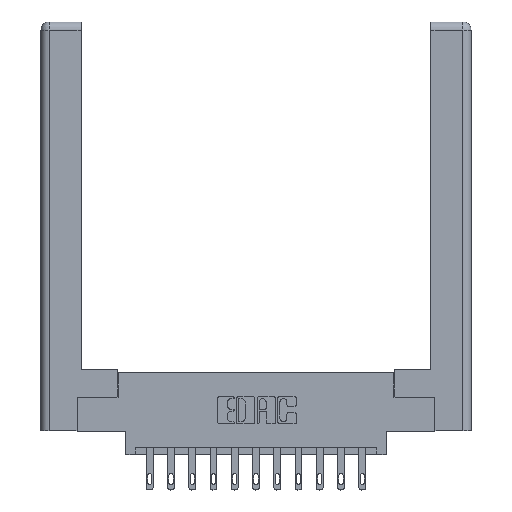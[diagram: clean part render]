
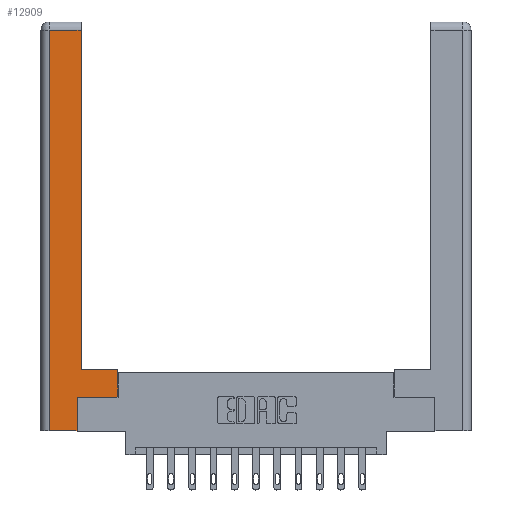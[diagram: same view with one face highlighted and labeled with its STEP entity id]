
A CAD part, top view. The second image highlights one B-rep face of the part: STEP entity #12909.
In plain terms, the highlighted planar face has unit normal (0, 0, 1).
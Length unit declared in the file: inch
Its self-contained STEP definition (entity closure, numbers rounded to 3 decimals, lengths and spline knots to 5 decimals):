
#191 = EDGE_CURVE ( 'NONE', #5089, #2664, #8265, .T. ) ;
#409 = CARTESIAN_POINT ( 'NONE',  ( 0.265, 0.245, 0. ) ) ;
#524 = CARTESIAN_POINT ( 'NONE',  ( 0.295, 2.94, 0. ) ) ;
#637 = DIRECTION ( 'NONE',  ( -1., 0., 0. ) ) ;
#660 = VECTOR ( 'NONE', #7658, 39.37008 ) ;
#1193 = VERTEX_POINT ( 'NONE', #10717 ) ;
#2319 = CARTESIAN_POINT ( 'NONE',  ( 0.565, 0.245, 0. ) ) ;
#2436 = VERTEX_POINT ( 'NONE', #524 ) ;
#2641 = DIRECTION ( 'NONE',  ( -1., 0., 0. ) ) ;
#2664 = VERTEX_POINT ( 'NONE', #14087 ) ;
#2863 = VECTOR ( 'NONE', #14801, 39.37008 ) ;
#3457 = EDGE_CURVE ( 'NONE', #7770, #2436, #3869, .T. ) ;
#3740 = CARTESIAN_POINT ( 'NONE',  ( 0.265, 0., 0. ) ) ;
#3869 = LINE ( 'NONE', #9389, #5882 ) ;
#4105 = EDGE_LOOP ( 'NONE', ( #7045, #4222, #13725, #10684, #13144, #4409, #6408, #6317 ) ) ;
#4153 = LINE ( 'NONE', #11201, #2863 ) ;
#4222 = ORIENTED_EDGE ( 'NONE', *, *, #10051, .T. ) ;
#4333 = EDGE_CURVE ( 'NONE', #14912, #11302, #10878, .T. ) ;
#4409 = ORIENTED_EDGE ( 'NONE', *, *, #7809, .T. ) ;
#4442 = DIRECTION ( 'NONE',  ( 0., 1., 0. ) ) ;
#4651 = VECTOR ( 'NONE', #6125, 39.37008 ) ;
#4731 = AXIS2_PLACEMENT_3D ( 'NONE', #11183, #9996, #637 ) ;
#4962 = CARTESIAN_POINT ( 'NONE',  ( 0.0615, 0., 0. ) ) ;
#4997 = CARTESIAN_POINT ( 'NONE',  ( 0.0615, 2.94, 0. ) ) ;
#5089 = VERTEX_POINT ( 'NONE', #9473 ) ;
#5126 = VECTOR ( 'NONE', #11988, 39.37008 ) ;
#5882 = VECTOR ( 'NONE', #10430, 39.37008 ) ;
#6070 = CARTESIAN_POINT ( 'NONE',  ( 0.295, 0.45, 0. ) ) ;
#6125 = DIRECTION ( 'NONE',  ( -1., 0., 0. ) ) ;
#6143 = LINE ( 'NONE', #2319, #7055 ) ;
#6317 = ORIENTED_EDGE ( 'NONE', *, *, #7481, .T. ) ;
#6408 = ORIENTED_EDGE ( 'NONE', *, *, #8894, .T. ) ;
#6705 = CARTESIAN_POINT ( 'NONE',  ( 0.265, 0.245, 0. ) ) ;
#6817 = VECTOR ( 'NONE', #4442, 39.37008 ) ;
#6964 = EDGE_CURVE ( 'NONE', #2664, #14912, #4153, .T. ) ;
#7045 = ORIENTED_EDGE ( 'NONE', *, *, #3457, .T. ) ;
#7055 = VECTOR ( 'NONE', #11638, 39.37008 ) ;
#7118 = VERTEX_POINT ( 'NONE', #11609 ) ;
#7481 = EDGE_CURVE ( 'NONE', #1193, #7770, #10954, .T. ) ;
#7658 = DIRECTION ( 'NONE',  ( 0., 1., 0. ) ) ;
#7667 = PLANE ( 'NONE',  #4731 ) ;
#7770 = VERTEX_POINT ( 'NONE', #13946 ) ;
#7809 = EDGE_CURVE ( 'NONE', #11302, #7118, #6143, .T. ) ;
#8265 = LINE ( 'NONE', #4962, #5126 ) ;
#8328 = LINE ( 'NONE', #4997, #4651 ) ;
#8623 = CARTESIAN_POINT ( 'NONE',  ( 0.565, 0.45, 0. ) ) ;
#8894 = EDGE_CURVE ( 'NONE', #7118, #1193, #13727, .T. ) ;
#9286 = VECTOR ( 'NONE', #2641, 39.37008 ) ;
#9389 = CARTESIAN_POINT ( 'NONE',  ( 0.295, 3., 0. ) ) ;
#9473 = CARTESIAN_POINT ( 'NONE',  ( 0.0615, 2.94, 0. ) ) ;
#9996 = DIRECTION ( 'NONE',  ( 0., 0., -1. ) ) ;
#10051 = EDGE_CURVE ( 'NONE', #2436, #5089, #8328, .T. ) ;
#10430 = DIRECTION ( 'NONE',  ( 0., 1., 0. ) ) ;
#10684 = ORIENTED_EDGE ( 'NONE', *, *, #6964, .T. ) ;
#10717 = CARTESIAN_POINT ( 'NONE',  ( 0.565, 0.45, 0. ) ) ;
#10878 = LINE ( 'NONE', #6705, #6817 ) ;
#10954 = LINE ( 'NONE', #6070, #9286 ) ;
#11183 = CARTESIAN_POINT ( 'NONE',  ( 0., 0., 0. ) ) ;
#11201 = CARTESIAN_POINT ( 'NONE',  ( 0.265, 0., 0. ) ) ;
#11302 = VERTEX_POINT ( 'NONE', #409 ) ;
#11609 = CARTESIAN_POINT ( 'NONE',  ( 0.565, 0.245, 0. ) ) ;
#11638 = DIRECTION ( 'NONE',  ( 1., 0., 0. ) ) ;
#11988 = DIRECTION ( 'NONE',  ( 0., -1., 0. ) ) ;
#12909 = ADVANCED_FACE ( 'NONE', ( #13324 ), #7667, .F. ) ;
#13144 = ORIENTED_EDGE ( 'NONE', *, *, #4333, .T. ) ;
#13324 = FACE_OUTER_BOUND ( 'NONE', #4105, .T. ) ;
#13725 = ORIENTED_EDGE ( 'NONE', *, *, #191, .T. ) ;
#13727 = LINE ( 'NONE', #8623, #660 ) ;
#13946 = CARTESIAN_POINT ( 'NONE',  ( 0.295, 0.45, 0. ) ) ;
#14087 = CARTESIAN_POINT ( 'NONE',  ( 0.0615, 0., 0. ) ) ;
#14801 = DIRECTION ( 'NONE',  ( 1., 0., 0. ) ) ;
#14912 = VERTEX_POINT ( 'NONE', #3740 ) ;
